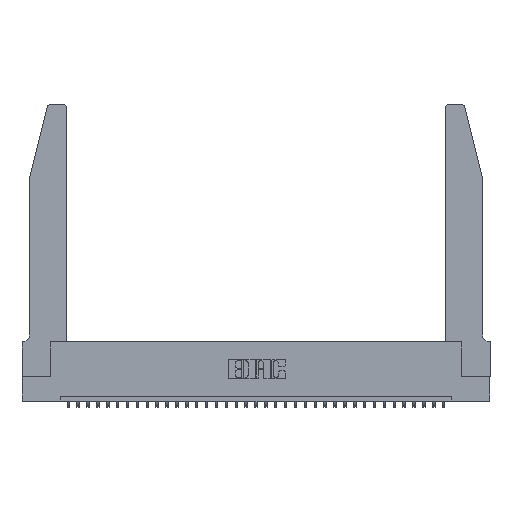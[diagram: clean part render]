
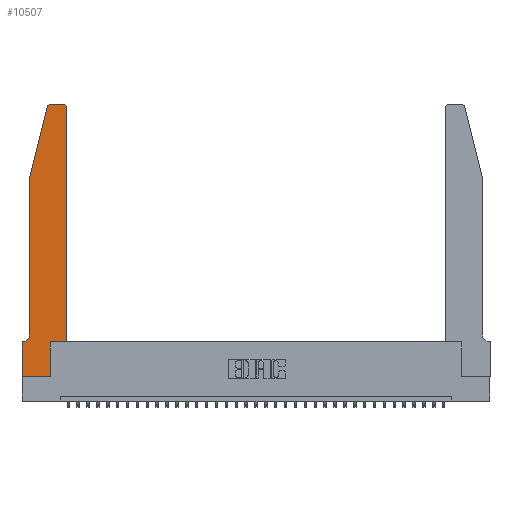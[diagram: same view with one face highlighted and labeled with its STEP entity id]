
A CAD part, top view. The second image highlights one B-rep face of the part: STEP entity #10507.
In plain terms, the highlighted planar face has unit normal (0, 0, 1).
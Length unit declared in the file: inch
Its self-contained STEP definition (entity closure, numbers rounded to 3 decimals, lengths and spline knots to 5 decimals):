
#60 = ORIENTED_EDGE ( 'NONE', *, *, #34152, .T. ) ;
#129 = VECTOR ( 'NONE', #27402, 39.37008 ) ;
#466 = CARTESIAN_POINT ( 'NONE',  ( 0.0055, 0.42, 0.37 ) ) ;
#475 = EDGE_LOOP ( 'NONE', ( #8445, #17922, #29666, #25223, #60, #27090, #31370, #27429, #11277, #5916, #32000, #1916 ) ) ;
#582 = DIRECTION ( 'NONE',  ( 0., -1., 0. ) ) ;
#1569 = LINE ( 'NONE', #6949, #32474 ) ;
#1578 = VERTEX_POINT ( 'NONE', #29951 ) ;
#1880 = VECTOR ( 'NONE', #4021, 39.37008 ) ;
#1916 = ORIENTED_EDGE ( 'NONE', *, *, #4315, .T. ) ;
#2764 = EDGE_CURVE ( 'NONE', #5678, #24921, #21903, .T. ) ;
#3348 = DIRECTION ( 'NONE',  ( -1., 0., 0. ) ) ;
#3415 = CARTESIAN_POINT ( 'NONE',  ( 0.0055, 0.35, 0.37 ) ) ;
#3550 = CARTESIAN_POINT ( 'NONE',  ( 0.4505, 0.35, 0.37 ) ) ;
#3578 = CARTESIAN_POINT ( 'NONE',  ( 0.2865, 0., 0.37 ) ) ;
#4021 = DIRECTION ( 'NONE',  ( 0., 1., 0. ) ) ;
#4315 = EDGE_CURVE ( 'NONE', #18599, #9963, #21423, .T. ) ;
#4516 = LINE ( 'NONE', #21542, #28795 ) ;
#4864 = VECTOR ( 'NONE', #32132, 39.37008 ) ;
#5269 = CARTESIAN_POINT ( 'NONE',  ( 0.4205, 2.72, 0.37 ) ) ;
#5678 = VERTEX_POINT ( 'NONE', #3415 ) ;
#5916 = ORIENTED_EDGE ( 'NONE', *, *, #8584, .T. ) ;
#6375 = CARTESIAN_POINT ( 'NONE',  ( 0.4505, 2.72, 0.37 ) ) ;
#6762 = CARTESIAN_POINT ( 'NONE',  ( 0., 0.35, 0.37 ) ) ;
#6882 = EDGE_CURVE ( 'NONE', #18658, #1578, #19141, .T. ) ;
#6949 = CARTESIAN_POINT ( 'NONE',  ( 0.2865, 0.35, 0.37 ) ) ;
#6955 = CARTESIAN_POINT ( 'NONE',  ( 0., 0., 0.37 ) ) ;
#7127 = VECTOR ( 'NONE', #3348, 39.37008 ) ;
#7210 = VERTEX_POINT ( 'NONE', #31644 ) ;
#7306 = EDGE_CURVE ( 'NONE', #1578, #20541, #8209, .T. ) ;
#7459 = CARTESIAN_POINT ( 'NONE',  ( 0.0755, 2., 0.37 ) ) ;
#7678 = VECTOR ( 'NONE', #12570, 39.37008 ) ;
#7682 = CARTESIAN_POINT ( 'NONE',  ( 0., 0.35, 0.37 ) ) ;
#7720 = VECTOR ( 'NONE', #582, 39.37008 ) ;
#7960 = DIRECTION ( 'NONE',  ( 0., 0., 1. ) ) ;
#8086 = DIRECTION ( 'NONE',  ( -1., 0., 0. ) ) ;
#8209 = LINE ( 'NONE', #7459, #4864 ) ;
#8398 = EDGE_CURVE ( 'NONE', #20541, #31473, #28995, .T. ) ;
#8445 = ORIENTED_EDGE ( 'NONE', *, *, #9029, .T. ) ;
#8584 = EDGE_CURVE ( 'NONE', #7210, #29521, #12257, .T. ) ;
#9029 = EDGE_CURVE ( 'NONE', #9963, #18658, #30616, .T. ) ;
#9278 = AXIS2_PLACEMENT_3D ( 'NONE', #7682, #29094, #13084 ) ;
#9963 = VERTEX_POINT ( 'NONE', #30403 ) ;
#10187 = CARTESIAN_POINT ( 'NONE',  ( 0.2605, 2.75, 0.37 ) ) ;
#10507 = ADVANCED_FACE ( 'NONE', ( #24647 ), #23729, .T. ) ;
#10664 = DIRECTION ( 'NONE',  ( 1., 0., 0. ) ) ;
#10675 = DIRECTION ( 'NONE',  ( 0., 0., -1. ) ) ;
#11277 = ORIENTED_EDGE ( 'NONE', *, *, #12462, .T. ) ;
#11718 = CARTESIAN_POINT ( 'NONE',  ( 0., 0., 0.37 ) ) ;
#11786 = EDGE_CURVE ( 'NONE', #27023, #27940, #4516, .T. ) ;
#12257 = LINE ( 'NONE', #15785, #13099 ) ;
#12462 = EDGE_CURVE ( 'NONE', #27940, #7210, #1569, .T. ) ;
#12570 = DIRECTION ( 'NONE',  ( -1., 0., 0. ) ) ;
#12867 = CARTESIAN_POINT ( 'NONE',  ( 0.0755, 2., 0.37 ) ) ;
#13084 = DIRECTION ( 'NONE',  ( 1., 0., 0. ) ) ;
#13099 = VECTOR ( 'NONE', #21122, 39.37008 ) ;
#13492 = AXIS2_PLACEMENT_3D ( 'NONE', #24530, #24422, #19284 ) ;
#14060 = DIRECTION ( 'NONE',  ( 1., 0., 0. ) ) ;
#14862 = LINE ( 'NONE', #3550, #1880 ) ;
#14872 = LINE ( 'NONE', #11718, #7720 ) ;
#15785 = CARTESIAN_POINT ( 'NONE',  ( 0.4505, 0.35, 0.37 ) ) ;
#17035 = AXIS2_PLACEMENT_3D ( 'NONE', #5269, #7960, #10664 ) ;
#17922 = ORIENTED_EDGE ( 'NONE', *, *, #6882, .T. ) ;
#18082 = CARTESIAN_POINT ( 'NONE',  ( 0.0755, 0.35, 0.37 ) ) ;
#18599 = VERTEX_POINT ( 'NONE', #6375 ) ;
#18658 = VERTEX_POINT ( 'NONE', #25282 ) ;
#18932 = EDGE_CURVE ( 'NONE', #29521, #18599, #14862, .T. ) ;
#19141 = CIRCLE ( 'NONE', #13492, 0.03 ) ;
#19232 = CARTESIAN_POINT ( 'NONE',  ( 0.0755, 2., 0.37 ) ) ;
#19284 = DIRECTION ( 'NONE',  ( 1., 0., 0. ) ) ;
#20541 = VERTEX_POINT ( 'NONE', #12867 ) ;
#21112 = CIRCLE ( 'NONE', #30237, 0.07 ) ;
#21122 = DIRECTION ( 'NONE',  ( 1., 0., 0. ) ) ;
#21423 = CIRCLE ( 'NONE', #17035, 0.03 ) ;
#21542 = CARTESIAN_POINT ( 'NONE',  ( 0., 0., 0.37 ) ) ;
#21903 = LINE ( 'NONE', #18082, #7678 ) ;
#23729 = PLANE ( 'NONE',  #9278 ) ;
#24422 = DIRECTION ( 'NONE',  ( 0., 0., 1. ) ) ;
#24530 = CARTESIAN_POINT ( 'NONE',  ( 0.284, 2.72, 0.37 ) ) ;
#24647 = FACE_OUTER_BOUND ( 'NONE', #475, .T. ) ;
#24921 = VERTEX_POINT ( 'NONE', #6762 ) ;
#25223 = ORIENTED_EDGE ( 'NONE', *, *, #8398, .T. ) ;
#25282 = CARTESIAN_POINT ( 'NONE',  ( 0.284, 2.75, 0.37 ) ) ;
#26202 = CARTESIAN_POINT ( 'NONE',  ( 0.4505, 0.35, 0.37 ) ) ;
#27023 = VERTEX_POINT ( 'NONE', #6955 ) ;
#27090 = ORIENTED_EDGE ( 'NONE', *, *, #2764, .T. ) ;
#27402 = DIRECTION ( 'NONE',  ( 0., -1., 0. ) ) ;
#27429 = ORIENTED_EDGE ( 'NONE', *, *, #11786, .T. ) ;
#27824 = CARTESIAN_POINT ( 'NONE',  ( 0.0755, 0.42, 0.37 ) ) ;
#27940 = VERTEX_POINT ( 'NONE', #3578 ) ;
#28795 = VECTOR ( 'NONE', #14060, 39.37008 ) ;
#28995 = LINE ( 'NONE', #19232, #129 ) ;
#29094 = DIRECTION ( 'NONE',  ( 0., 0., 1. ) ) ;
#29521 = VERTEX_POINT ( 'NONE', #26202 ) ;
#29666 = ORIENTED_EDGE ( 'NONE', *, *, #7306, .T. ) ;
#29951 = CARTESIAN_POINT ( 'NONE',  ( 0.25487, 2.72718, 0.37 ) ) ;
#30237 = AXIS2_PLACEMENT_3D ( 'NONE', #466, #10675, #8086 ) ;
#30403 = CARTESIAN_POINT ( 'NONE',  ( 0.4205, 2.75, 0.37 ) ) ;
#30616 = LINE ( 'NONE', #10187, #7127 ) ;
#31370 = ORIENTED_EDGE ( 'NONE', *, *, #34228, .T. ) ;
#31473 = VERTEX_POINT ( 'NONE', #27824 ) ;
#31644 = CARTESIAN_POINT ( 'NONE',  ( 0.2865, 0.35, 0.37 ) ) ;
#32000 = ORIENTED_EDGE ( 'NONE', *, *, #18932, .T. ) ;
#32132 = DIRECTION ( 'NONE',  ( -0.239, -0.971, 0. ) ) ;
#32474 = VECTOR ( 'NONE', #33877, 39.37008 ) ;
#33877 = DIRECTION ( 'NONE',  ( 0., 1., 0. ) ) ;
#34152 = EDGE_CURVE ( 'NONE', #31473, #5678, #21112, .T. ) ;
#34228 = EDGE_CURVE ( 'NONE', #24921, #27023, #14872, .T. ) ;
